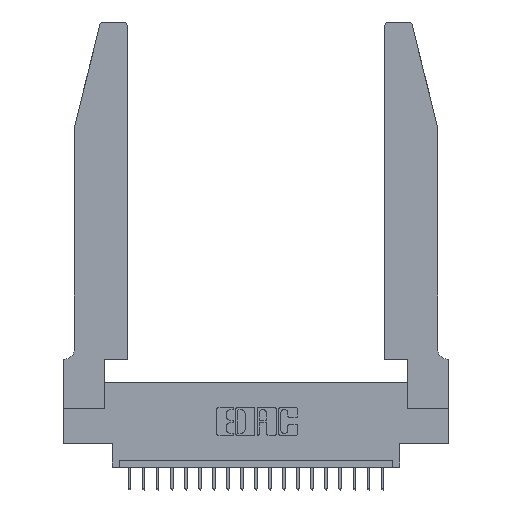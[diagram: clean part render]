
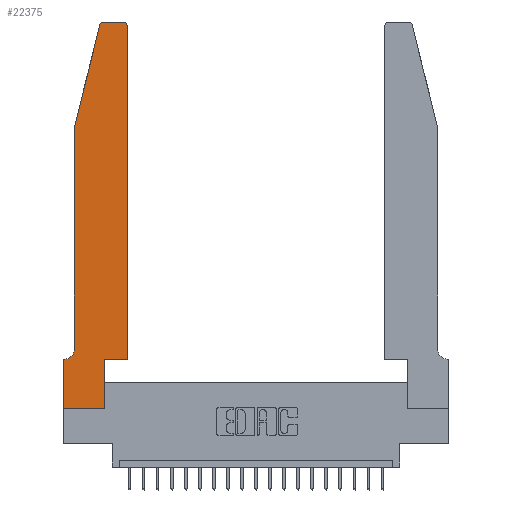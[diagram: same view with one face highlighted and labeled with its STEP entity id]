
A CAD part, top view. The second image highlights one B-rep face of the part: STEP entity #22375.
In plain terms, the highlighted planar face has unit normal (0, 0, 1).
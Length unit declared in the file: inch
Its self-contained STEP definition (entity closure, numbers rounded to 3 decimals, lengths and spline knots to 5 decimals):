
#93 = EDGE_CURVE ( 'NONE', #14853, #3309, #2532, .T. ) ;
#179 = CIRCLE ( 'NONE', #19690, 0.03 ) ;
#220 = AXIS2_PLACEMENT_3D ( 'NONE', #5989, #4265, #13098 ) ;
#306 = EDGE_CURVE ( 'NONE', #13835, #22331, #5213, .T. ) ;
#382 = DIRECTION ( 'NONE',  ( 1., 0., 0. ) ) ;
#469 = ORIENTED_EDGE ( 'NONE', *, *, #10085, .T. ) ;
#876 = VERTEX_POINT ( 'NONE', #5700 ) ;
#1675 = DIRECTION ( 'NONE',  ( -1., 0., 0. ) ) ;
#1698 = DIRECTION ( 'NONE',  ( 0., 1., 0. ) ) ;
#2000 = EDGE_CURVE ( 'NONE', #5381, #22332, #18956, .T. ) ;
#2306 = CARTESIAN_POINT ( 'NONE',  ( 0.284, 2.72, 0.37 ) ) ;
#2413 = PLANE ( 'NONE',  #18895 ) ;
#2486 = CARTESIAN_POINT ( 'NONE',  ( 0.2865, 0., 0.37 ) ) ;
#2532 = CIRCLE ( 'NONE', #220, 0.03 ) ;
#2623 = LINE ( 'NONE', #9549, #20764 ) ;
#2973 = DIRECTION ( 'NONE',  ( 0., 0., 1. ) ) ;
#3189 = VECTOR ( 'NONE', #7080, 39.37008 ) ;
#3261 = LINE ( 'NONE', #3443, #7319 ) ;
#3309 = VERTEX_POINT ( 'NONE', #4514 ) ;
#3443 = CARTESIAN_POINT ( 'NONE',  ( 0.0755, 2., 0.37 ) ) ;
#3497 = LINE ( 'NONE', #16052, #3747 ) ;
#3602 = CARTESIAN_POINT ( 'NONE',  ( 0.2865, 0.35, 0.37 ) ) ;
#3647 = CIRCLE ( 'NONE', #7449, 0.07 ) ;
#3747 = VECTOR ( 'NONE', #21229, 39.37008 ) ;
#3791 = CARTESIAN_POINT ( 'NONE',  ( 0.25487, 2.72718, 0.37 ) ) ;
#4139 = DIRECTION ( 'NONE',  ( 0., 0., 1. ) ) ;
#4162 = ORIENTED_EDGE ( 'NONE', *, *, #11780, .T. ) ;
#4265 = DIRECTION ( 'NONE',  ( 0., 0., 1. ) ) ;
#4391 = VERTEX_POINT ( 'NONE', #12725 ) ;
#4432 = EDGE_CURVE ( 'NONE', #3309, #876, #2623, .T. ) ;
#4514 = CARTESIAN_POINT ( 'NONE',  ( 0.4205, 2.75, 0.37 ) ) ;
#4923 = LINE ( 'NONE', #10547, #6556 ) ;
#5213 = LINE ( 'NONE', #17552, #12250 ) ;
#5381 = VERTEX_POINT ( 'NONE', #16326 ) ;
#5470 = DIRECTION ( 'NONE',  ( -1., 0., 0. ) ) ;
#5700 = CARTESIAN_POINT ( 'NONE',  ( 0.284, 2.75, 0.37 ) ) ;
#5989 = CARTESIAN_POINT ( 'NONE',  ( 0.4205, 2.72, 0.37 ) ) ;
#6556 = VECTOR ( 'NONE', #1698, 39.37008 ) ;
#6620 = VECTOR ( 'NONE', #10964, 39.37008 ) ;
#6917 = EDGE_CURVE ( 'NONE', #22331, #5381, #10243, .T. ) ;
#7080 = DIRECTION ( 'NONE',  ( 0., 1., 0. ) ) ;
#7293 = DIRECTION ( 'NONE',  ( 0., 0., -1. ) ) ;
#7319 = VECTOR ( 'NONE', #12438, 39.37008 ) ;
#7449 = AXIS2_PLACEMENT_3D ( 'NONE', #11999, #7293, #5470 ) ;
#7708 = LINE ( 'NONE', #12922, #6620 ) ;
#7955 = VECTOR ( 'NONE', #1675, 39.37008 ) ;
#8251 = ORIENTED_EDGE ( 'NONE', *, *, #20936, .T. ) ;
#8696 = CARTESIAN_POINT ( 'NONE',  ( 0.4505, 2.72, 0.37 ) ) ;
#8754 = EDGE_CURVE ( 'NONE', #4391, #20998, #7708, .T. ) ;
#8976 = EDGE_CURVE ( 'NONE', #20998, #20372, #3647, .T. ) ;
#9436 = CARTESIAN_POINT ( 'NONE',  ( 0.4505, 0.35, 0.37 ) ) ;
#9516 = DIRECTION ( 'NONE',  ( 1., 0., 0. ) ) ;
#9549 = CARTESIAN_POINT ( 'NONE',  ( 0.2605, 2.75, 0.37 ) ) ;
#9582 = VERTEX_POINT ( 'NONE', #13367 ) ;
#10085 = EDGE_CURVE ( 'NONE', #22332, #14853, #4923, .T. ) ;
#10243 = LINE ( 'NONE', #3602, #3189 ) ;
#10343 = ORIENTED_EDGE ( 'NONE', *, *, #6917, .T. ) ;
#10547 = CARTESIAN_POINT ( 'NONE',  ( 0.4505, 0.35, 0.37 ) ) ;
#10564 = CARTESIAN_POINT ( 'NONE',  ( 0.0755, 0.42, 0.37 ) ) ;
#10964 = DIRECTION ( 'NONE',  ( 0., -1., 0. ) ) ;
#11108 = CARTESIAN_POINT ( 'NONE',  ( 0., 0.35, 0.37 ) ) ;
#11780 = EDGE_CURVE ( 'NONE', #9582, #13835, #3497, .T. ) ;
#11913 = VECTOR ( 'NONE', #13336, 39.37008 ) ;
#11948 = CARTESIAN_POINT ( 'NONE',  ( 0.0055, 0.35, 0.37 ) ) ;
#11999 = CARTESIAN_POINT ( 'NONE',  ( 0.0055, 0.42, 0.37 ) ) ;
#12157 = ORIENTED_EDGE ( 'NONE', *, *, #8976, .T. ) ;
#12250 = VECTOR ( 'NONE', #382, 39.37008 ) ;
#12438 = DIRECTION ( 'NONE',  ( -0.239, -0.971, 0. ) ) ;
#12725 = CARTESIAN_POINT ( 'NONE',  ( 0.0755, 2., 0.37 ) ) ;
#12814 = ORIENTED_EDGE ( 'NONE', *, *, #14810, .T. ) ;
#12922 = CARTESIAN_POINT ( 'NONE',  ( 0.0755, 2., 0.37 ) ) ;
#13098 = DIRECTION ( 'NONE',  ( 1., 0., 0. ) ) ;
#13336 = DIRECTION ( 'NONE',  ( 1., 0., 0. ) ) ;
#13367 = CARTESIAN_POINT ( 'NONE',  ( 0., 0.35, 0.37 ) ) ;
#13678 = EDGE_CURVE ( 'NONE', #876, #13928, #179, .T. ) ;
#13835 = VERTEX_POINT ( 'NONE', #22234 ) ;
#13928 = VERTEX_POINT ( 'NONE', #3791 ) ;
#14647 = FACE_OUTER_BOUND ( 'NONE', #15646, .T. ) ;
#14810 = EDGE_CURVE ( 'NONE', #20372, #9582, #20168, .T. ) ;
#14853 = VERTEX_POINT ( 'NONE', #8696 ) ;
#15143 = ORIENTED_EDGE ( 'NONE', *, *, #4432, .T. ) ;
#15646 = EDGE_LOOP ( 'NONE', ( #15143, #22263, #8251, #22285, #12157, #12814, #4162, #18657, #10343, #16881, #469, #20542 ) ) ;
#16052 = CARTESIAN_POINT ( 'NONE',  ( 0., 0., 0.37 ) ) ;
#16326 = CARTESIAN_POINT ( 'NONE',  ( 0.2865, 0.35, 0.37 ) ) ;
#16881 = ORIENTED_EDGE ( 'NONE', *, *, #2000, .T. ) ;
#17347 = CARTESIAN_POINT ( 'NONE',  ( 0.0755, 0.35, 0.37 ) ) ;
#17552 = CARTESIAN_POINT ( 'NONE',  ( 0., 0., 0.37 ) ) ;
#18112 = DIRECTION ( 'NONE',  ( -1., 0., 0. ) ) ;
#18657 = ORIENTED_EDGE ( 'NONE', *, *, #306, .T. ) ;
#18895 = AXIS2_PLACEMENT_3D ( 'NONE', #11108, #4139, #9516 ) ;
#18956 = LINE ( 'NONE', #20249, #11913 ) ;
#19690 = AXIS2_PLACEMENT_3D ( 'NONE', #2306, #2973, #20646 ) ;
#20168 = LINE ( 'NONE', #17347, #7955 ) ;
#20249 = CARTESIAN_POINT ( 'NONE',  ( 0.4505, 0.35, 0.37 ) ) ;
#20372 = VERTEX_POINT ( 'NONE', #11948 ) ;
#20542 = ORIENTED_EDGE ( 'NONE', *, *, #93, .T. ) ;
#20646 = DIRECTION ( 'NONE',  ( 1., 0., 0. ) ) ;
#20764 = VECTOR ( 'NONE', #18112, 39.37008 ) ;
#20936 = EDGE_CURVE ( 'NONE', #13928, #4391, #3261, .T. ) ;
#20998 = VERTEX_POINT ( 'NONE', #10564 ) ;
#21229 = DIRECTION ( 'NONE',  ( 0., -1., 0. ) ) ;
#22234 = CARTESIAN_POINT ( 'NONE',  ( 0., 0., 0.37 ) ) ;
#22263 = ORIENTED_EDGE ( 'NONE', *, *, #13678, .T. ) ;
#22285 = ORIENTED_EDGE ( 'NONE', *, *, #8754, .T. ) ;
#22331 = VERTEX_POINT ( 'NONE', #2486 ) ;
#22332 = VERTEX_POINT ( 'NONE', #9436 ) ;
#22375 = ADVANCED_FACE ( 'NONE', ( #14647 ), #2413, .T. ) ;
